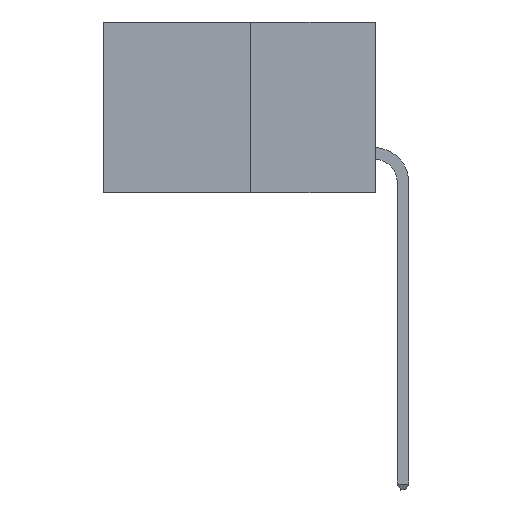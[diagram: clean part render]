
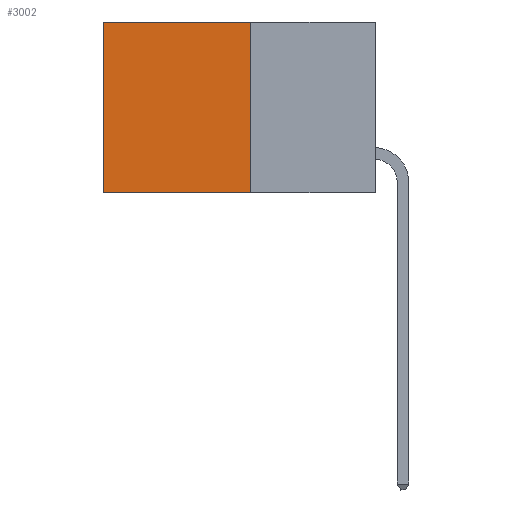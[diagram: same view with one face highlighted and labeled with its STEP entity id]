
A CAD part, left-side view. The second image highlights one B-rep face of the part: STEP entity #3002.
In plain terms, the highlighted planar face has unit normal (-1, 0, 0).
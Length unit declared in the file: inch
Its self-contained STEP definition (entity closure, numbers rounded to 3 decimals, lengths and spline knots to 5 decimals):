
#64 = VECTOR ( 'NONE', #11748, 39.37008 ) ;
#725 = VECTOR ( 'NONE', #15667, 39.37008 ) ;
#763 = DIRECTION ( 'NONE',  ( 1., 0., 0. ) ) ;
#958 = LINE ( 'NONE', #10550, #64 ) ;
#1946 = LINE ( 'NONE', #14304, #8249 ) ;
#1957 = DIRECTION ( 'NONE',  ( 0., 0., -1. ) ) ;
#3002 = ADVANCED_FACE ( 'NONE', ( #14947 ), #15562, .F. ) ;
#3157 = EDGE_LOOP ( 'NONE', ( #11225, #10905, #14983, #14660 ) ) ;
#4472 = VECTOR ( 'NONE', #11591, 39.37008 ) ;
#5197 = VERTEX_POINT ( 'NONE', #6228 ) ;
#5627 = EDGE_CURVE ( 'NONE', #11157, #9745, #1946, .T. ) ;
#6228 = CARTESIAN_POINT ( 'NONE',  ( 0.277, 0.59, -0.37 ) ) ;
#7519 = EDGE_CURVE ( 'NONE', #13674, #5197, #958, .T. ) ;
#8159 = CARTESIAN_POINT ( 'NONE',  ( 0.277, 0.27, -0.37 ) ) ;
#8249 = VECTOR ( 'NONE', #1957, 39.37008 ) ;
#8481 = CARTESIAN_POINT ( 'NONE',  ( 0.277, 0.27, 0. ) ) ;
#9584 = DIRECTION ( 'NONE',  ( 0., 0., -1. ) ) ;
#9745 = VERTEX_POINT ( 'NONE', #8159 ) ;
#9908 = CARTESIAN_POINT ( 'NONE',  ( 0.277, 0.59, 0. ) ) ;
#10391 = CARTESIAN_POINT ( 'NONE',  ( 0.277, 0.27, -0.37 ) ) ;
#10550 = CARTESIAN_POINT ( 'NONE',  ( 0.277, 0.59, -0.37 ) ) ;
#10905 = ORIENTED_EDGE ( 'NONE', *, *, #13169, .F. ) ;
#11157 = VERTEX_POINT ( 'NONE', #13000 ) ;
#11225 = ORIENTED_EDGE ( 'NONE', *, *, #7519, .T. ) ;
#11274 = EDGE_CURVE ( 'NONE', #11157, #13674, #13594, .T. ) ;
#11591 = DIRECTION ( 'NONE',  ( 0., 1., 0. ) ) ;
#11748 = DIRECTION ( 'NONE',  ( 0., 0., -1. ) ) ;
#13000 = CARTESIAN_POINT ( 'NONE',  ( 0.277, 0.27, 0. ) ) ;
#13169 = EDGE_CURVE ( 'NONE', #9745, #5197, #14205, .T. ) ;
#13594 = LINE ( 'NONE', #8481, #725 ) ;
#13674 = VERTEX_POINT ( 'NONE', #9908 ) ;
#14205 = LINE ( 'NONE', #10391, #4472 ) ;
#14304 = CARTESIAN_POINT ( 'NONE',  ( 0.277, 0.27, -0.37 ) ) ;
#14660 = ORIENTED_EDGE ( 'NONE', *, *, #11274, .T. ) ;
#14947 = FACE_OUTER_BOUND ( 'NONE', #3157, .T. ) ;
#14952 = AXIS2_PLACEMENT_3D ( 'NONE', #15523, #763, #9584 ) ;
#14983 = ORIENTED_EDGE ( 'NONE', *, *, #5627, .F. ) ;
#15523 = CARTESIAN_POINT ( 'NONE',  ( 0.277, 0.27, -0.37 ) ) ;
#15562 = PLANE ( 'NONE',  #14952 ) ;
#15667 = DIRECTION ( 'NONE',  ( 0., 1., 0. ) ) ;
